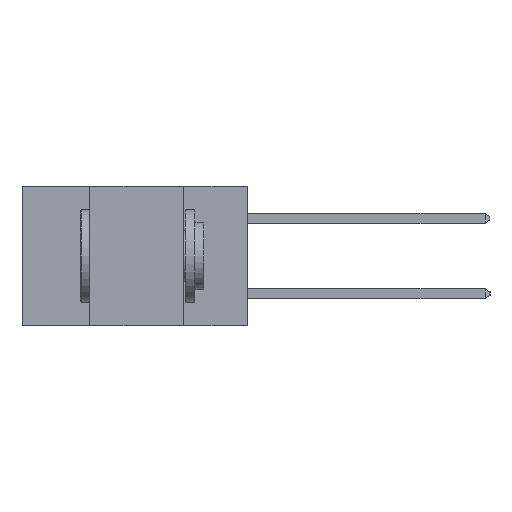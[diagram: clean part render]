
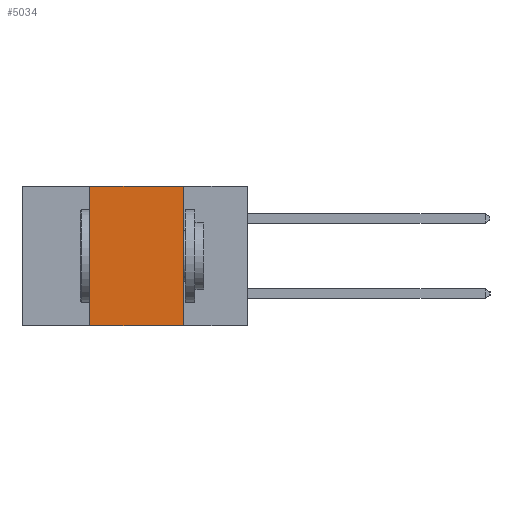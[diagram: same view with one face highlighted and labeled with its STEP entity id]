
A CAD part, left-side view. The second image highlights one B-rep face of the part: STEP entity #5034.
In plain terms, the highlighted planar face has unit normal (-1, 0, 0).
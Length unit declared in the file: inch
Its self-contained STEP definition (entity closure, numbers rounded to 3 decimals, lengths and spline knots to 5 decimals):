
#195 = DIRECTION ( 'NONE',  ( 0., 0., -1. ) ) ;
#2340 = EDGE_CURVE ( 'NONE', #23792, #12079, #9696, .T. ) ;
#2956 = CARTESIAN_POINT ( 'NONE',  ( 0., 0.6, -0.37 ) ) ;
#3413 = VECTOR ( 'NONE', #195, 39.37008 ) ;
#3723 = VECTOR ( 'NONE', #21742, 39.37008 ) ;
#4187 = ORIENTED_EDGE ( 'NONE', *, *, #26740, .T. ) ;
#5034 = ADVANCED_FACE ( 'NONE', ( #26011 ), #6932, .F. ) ;
#5521 = CARTESIAN_POINT ( 'NONE',  ( 0., 0.17, 0. ) ) ;
#5879 = CARTESIAN_POINT ( 'NONE',  ( 0., 0.17, -0.37 ) ) ;
#5917 = CARTESIAN_POINT ( 'NONE',  ( 0., 0.42, -0.37 ) ) ;
#6844 = DIRECTION ( 'NONE',  ( 0., 0., -1. ) ) ;
#6850 = DIRECTION ( 'NONE',  ( 1., 0., 0. ) ) ;
#6881 = CARTESIAN_POINT ( 'NONE',  ( 0., 0.6, 0. ) ) ;
#6932 = PLANE ( 'NONE',  #22023 ) ;
#7718 = VERTEX_POINT ( 'NONE', #26450 ) ;
#8162 = DIRECTION ( 'NONE',  ( 0., 0., 1. ) ) ;
#9207 = CARTESIAN_POINT ( 'NONE',  ( 0., 0.17, -0.37 ) ) ;
#9696 = LINE ( 'NONE', #9207, #3413 ) ;
#12079 = VERTEX_POINT ( 'NONE', #5879 ) ;
#12080 = CARTESIAN_POINT ( 'NONE',  ( 0., 0.42, -0.37 ) ) ;
#12471 = LINE ( 'NONE', #5917, #17370 ) ;
#13468 = VERTEX_POINT ( 'NONE', #12080 ) ;
#15349 = ORIENTED_EDGE ( 'NONE', *, *, #19841, .F. ) ;
#16838 = EDGE_CURVE ( 'NONE', #7718, #23792, #25325, .T. ) ;
#17370 = VECTOR ( 'NONE', #8162, 39.37008 ) ;
#19841 = EDGE_CURVE ( 'NONE', #13468, #7718, #12471, .T. ) ;
#20047 = VECTOR ( 'NONE', #23011, 39.37008 ) ;
#20404 = LINE ( 'NONE', #2956, #3723 ) ;
#21016 = CARTESIAN_POINT ( 'NONE',  ( 0., 0.6, 0. ) ) ;
#21461 = ORIENTED_EDGE ( 'NONE', *, *, #16838, .F. ) ;
#21742 = DIRECTION ( 'NONE',  ( 0., -1., 0. ) ) ;
#22023 = AXIS2_PLACEMENT_3D ( 'NONE', #6881, #6850, #6844 ) ;
#23011 = DIRECTION ( 'NONE',  ( 0., -1., 0. ) ) ;
#23792 = VERTEX_POINT ( 'NONE', #5521 ) ;
#24184 = EDGE_LOOP ( 'NONE', ( #26732, #21461, #15349, #4187 ) ) ;
#25325 = LINE ( 'NONE', #21016, #20047 ) ;
#26011 = FACE_OUTER_BOUND ( 'NONE', #24184, .T. ) ;
#26450 = CARTESIAN_POINT ( 'NONE',  ( 0., 0.42, 0. ) ) ;
#26732 = ORIENTED_EDGE ( 'NONE', *, *, #2340, .F. ) ;
#26740 = EDGE_CURVE ( 'NONE', #13468, #12079, #20404, .T. ) ;
